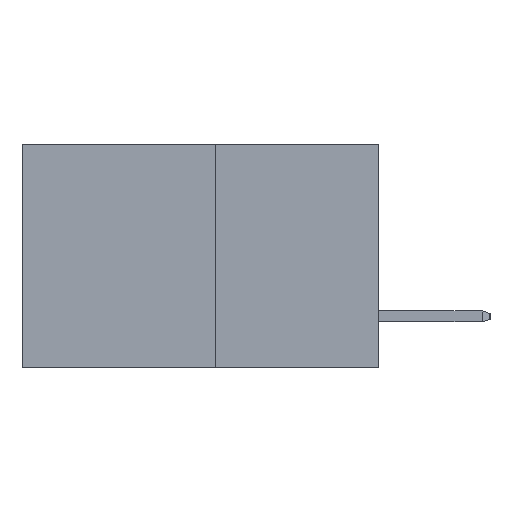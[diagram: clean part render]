
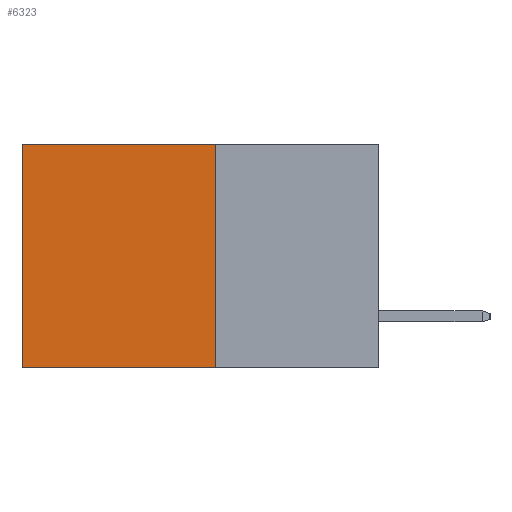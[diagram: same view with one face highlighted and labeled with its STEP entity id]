
A CAD part, left-side view. The second image highlights one B-rep face of the part: STEP entity #6323.
In plain terms, the highlighted planar face has unit normal (-1, 0, 0).
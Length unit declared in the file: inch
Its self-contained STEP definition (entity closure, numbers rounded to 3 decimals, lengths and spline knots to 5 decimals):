
#26 = AXIS2_PLACEMENT_3D ( 'NONE', #347, #217, #208 ) ;
#208 = DIRECTION ( 'NONE',  ( 0., 0., -1. ) ) ;
#217 = DIRECTION ( 'NONE',  ( 1., 0., 0. ) ) ;
#242 = PLANE ( 'NONE',  #26 ) ;
#347 = CARTESIAN_POINT ( 'NONE',  ( 0.277, 0.27, -0.37 ) ) ;
#427 = CARTESIAN_POINT ( 'NONE',  ( 0.277, 0.27, -0.37 ) ) ;
#864 = VECTOR ( 'NONE', #13945, 39.37008 ) ;
#1017 = EDGE_CURVE ( 'NONE', #1466, #1051, #13899, .T. ) ;
#1051 = VERTEX_POINT ( 'NONE', #9359 ) ;
#1466 = VERTEX_POINT ( 'NONE', #13559 ) ;
#1539 = VECTOR ( 'NONE', #5743, 39.37008 ) ;
#1753 = VERTEX_POINT ( 'NONE', #14119 ) ;
#1910 = CARTESIAN_POINT ( 'NONE',  ( 0.277, 0.27, 0. ) ) ;
#2963 = VECTOR ( 'NONE', #4304, 39.37008 ) ;
#4010 = EDGE_CURVE ( 'NONE', #1753, #9454, #10165, .T. ) ;
#4304 = DIRECTION ( 'NONE',  ( 0., 1., 0. ) ) ;
#4818 = VECTOR ( 'NONE', #9512, 39.37008 ) ;
#5606 = FACE_OUTER_BOUND ( 'NONE', #12692, .T. ) ;
#5743 = DIRECTION ( 'NONE',  ( 0., 0., -1. ) ) ;
#5824 = CARTESIAN_POINT ( 'NONE',  ( 0.277, 0.27, -0.37 ) ) ;
#6063 = LINE ( 'NONE', #1910, #2963 ) ;
#6323 = ADVANCED_FACE ( 'NONE', ( #5606 ), #242, .F. ) ;
#6462 = ORIENTED_EDGE ( 'NONE', *, *, #1017, .T. ) ;
#8099 = ORIENTED_EDGE ( 'NONE', *, *, #8514, .F. ) ;
#8514 = EDGE_CURVE ( 'NONE', #9454, #1051, #10255, .T. ) ;
#9324 = ORIENTED_EDGE ( 'NONE', *, *, #14104, .T. ) ;
#9359 = CARTESIAN_POINT ( 'NONE',  ( 0.277, 0.59, -0.37 ) ) ;
#9454 = VERTEX_POINT ( 'NONE', #427 ) ;
#9512 = DIRECTION ( 'NONE',  ( 0., 0., -1. ) ) ;
#10103 = CARTESIAN_POINT ( 'NONE',  ( 0.277, 0.59, -0.37 ) ) ;
#10165 = LINE ( 'NONE', #5824, #1539 ) ;
#10219 = ORIENTED_EDGE ( 'NONE', *, *, #4010, .F. ) ;
#10255 = LINE ( 'NONE', #12802, #864 ) ;
#12692 = EDGE_LOOP ( 'NONE', ( #6462, #8099, #10219, #9324 ) ) ;
#12802 = CARTESIAN_POINT ( 'NONE',  ( 0.277, 0.27, -0.37 ) ) ;
#13559 = CARTESIAN_POINT ( 'NONE',  ( 0.277, 0.59, 0. ) ) ;
#13899 = LINE ( 'NONE', #10103, #4818 ) ;
#13945 = DIRECTION ( 'NONE',  ( 0., 1., 0. ) ) ;
#14104 = EDGE_CURVE ( 'NONE', #1753, #1466, #6063, .T. ) ;
#14119 = CARTESIAN_POINT ( 'NONE',  ( 0.277, 0.27, 0. ) ) ;
